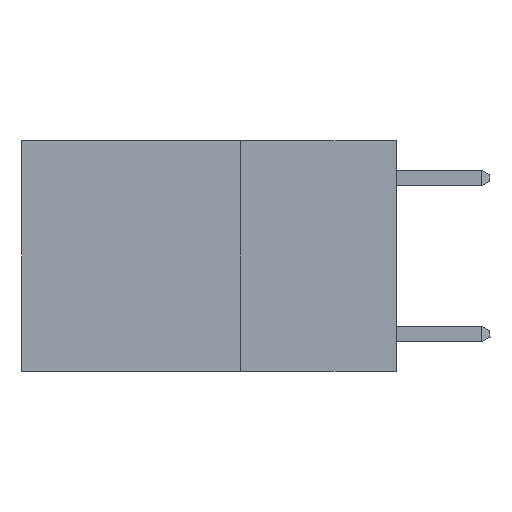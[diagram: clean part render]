
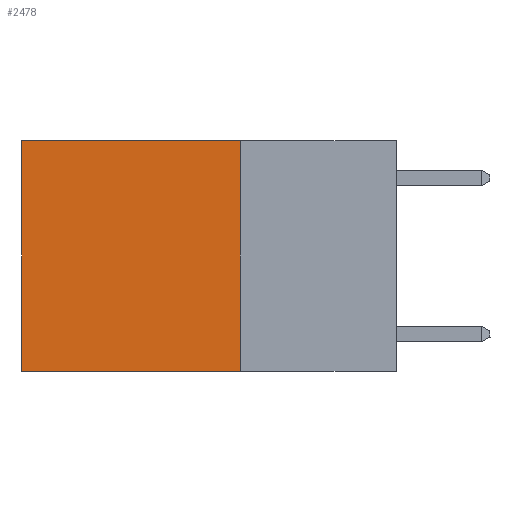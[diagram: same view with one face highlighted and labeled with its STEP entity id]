
A CAD part, left-side view. The second image highlights one B-rep face of the part: STEP entity #2478.
In plain terms, the highlighted planar face has unit normal (-1, 0, 0).
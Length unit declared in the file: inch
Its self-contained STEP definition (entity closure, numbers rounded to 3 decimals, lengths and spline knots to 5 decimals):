
#181 = FACE_OUTER_BOUND ( 'NONE', #15245, .T. ) ;
#490 = VERTEX_POINT ( 'NONE', #13582 ) ;
#2478 = ADVANCED_FACE ( 'NONE', ( #181 ), #11829, .F. ) ;
#2750 = AXIS2_PLACEMENT_3D ( 'NONE', #13504, #15144, #4949 ) ;
#3527 = CARTESIAN_POINT ( 'NONE',  ( 0.2625, 0.6, -0.37 ) ) ;
#3559 = ORIENTED_EDGE ( 'NONE', *, *, #11797, .F. ) ;
#4753 = DIRECTION ( 'NONE',  ( 0., 0., -1. ) ) ;
#4896 = ORIENTED_EDGE ( 'NONE', *, *, #14787, .F. ) ;
#4949 = DIRECTION ( 'NONE',  ( 0., 0., -1. ) ) ;
#4968 = CARTESIAN_POINT ( 'NONE',  ( 0.2625, 0.25, 0. ) ) ;
#5818 = VERTEX_POINT ( 'NONE', #3527 ) ;
#6146 = CARTESIAN_POINT ( 'NONE',  ( 0.2625, 0.25, 0. ) ) ;
#6965 = EDGE_CURVE ( 'NONE', #8553, #15794, #17427, .T. ) ;
#6987 = DIRECTION ( 'NONE',  ( 0., 1., 0. ) ) ;
#8553 = VERTEX_POINT ( 'NONE', #4968 ) ;
#8621 = EDGE_CURVE ( 'NONE', #15794, #5818, #9225, .T. ) ;
#9119 = VECTOR ( 'NONE', #13746, 39.37008 ) ;
#9225 = LINE ( 'NONE', #15389, #9119 ) ;
#9631 = DIRECTION ( 'NONE',  ( 0., 1., 0. ) ) ;
#11797 = EDGE_CURVE ( 'NONE', #490, #5818, #12374, .T. ) ;
#11829 = PLANE ( 'NONE',  #2750 ) ;
#12060 = VECTOR ( 'NONE', #6987, 39.37008 ) ;
#12374 = LINE ( 'NONE', #16965, #12060 ) ;
#12491 = CARTESIAN_POINT ( 'NONE',  ( 0.2625, 0.6, 0. ) ) ;
#12724 = ORIENTED_EDGE ( 'NONE', *, *, #6965, .T. ) ;
#12812 = ORIENTED_EDGE ( 'NONE', *, *, #8621, .T. ) ;
#13504 = CARTESIAN_POINT ( 'NONE',  ( 0.2625, 0.25, 0. ) ) ;
#13582 = CARTESIAN_POINT ( 'NONE',  ( 0.2625, 0.25, -0.37 ) ) ;
#13746 = DIRECTION ( 'NONE',  ( 0., 0., -1. ) ) ;
#14787 = EDGE_CURVE ( 'NONE', #8553, #490, #20184, .T. ) ;
#15144 = DIRECTION ( 'NONE',  ( 1., 0., 0. ) ) ;
#15245 = EDGE_LOOP ( 'NONE', ( #12812, #3559, #4896, #12724 ) ) ;
#15389 = CARTESIAN_POINT ( 'NONE',  ( 0.2625, 0.6, 0. ) ) ;
#15794 = VERTEX_POINT ( 'NONE', #12491 ) ;
#16581 = CARTESIAN_POINT ( 'NONE',  ( 0.2625, 0.25, 0. ) ) ;
#16965 = CARTESIAN_POINT ( 'NONE',  ( 0.2625, 0.25, -0.37 ) ) ;
#17346 = VECTOR ( 'NONE', #9631, 39.37008 ) ;
#17427 = LINE ( 'NONE', #6146, #17346 ) ;
#19211 = VECTOR ( 'NONE', #4753, 39.37008 ) ;
#20184 = LINE ( 'NONE', #16581, #19211 ) ;
